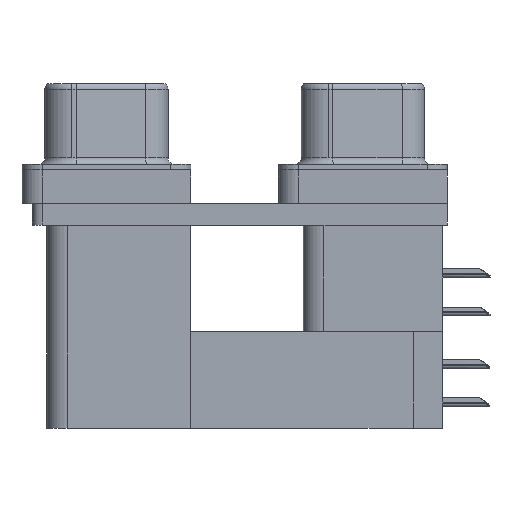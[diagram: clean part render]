
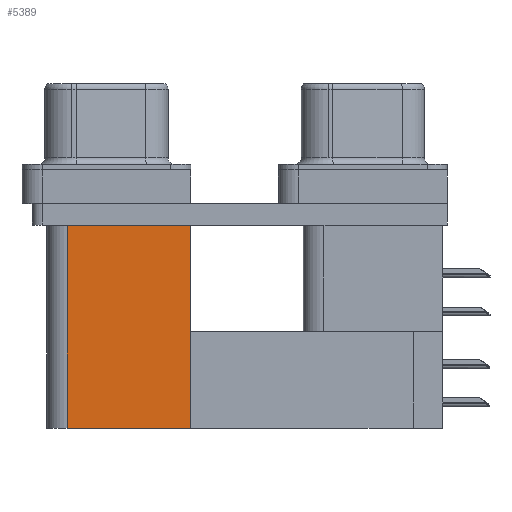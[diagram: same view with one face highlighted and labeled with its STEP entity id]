
A CAD part, left-side view. The second image highlights one B-rep face of the part: STEP entity #5389.
In plain terms, the highlighted planar face has unit normal (-1, 0, 0).
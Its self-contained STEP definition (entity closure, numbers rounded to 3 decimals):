
#396 = DIRECTION ( 'NONE',  ( 0., 1., 0. ) ) ;
#491 = PLANE ( 'NONE',  #10745 ) ;
#2394 = LINE ( 'NONE', #20965, #33138 ) ;
#3952 = ORIENTED_EDGE ( 'NONE', *, *, #31224, .F. ) ;
#5066 = FACE_OUTER_BOUND ( 'NONE', #18854, .T. ) ;
#5213 = VERTEX_POINT ( 'NONE', #20156 ) ;
#5389 = ADVANCED_FACE ( 'NONE', ( #5066 ), #491, .F. ) ;
#5781 = CARTESIAN_POINT ( 'NONE',  ( 3.7, 12.775, -19.2 ) ) ;
#6818 = ORIENTED_EDGE ( 'NONE', *, *, #19897, .T. ) ;
#6927 = CARTESIAN_POINT ( 'NONE',  ( 3.7, 21.975, -2.5 ) ) ;
#10745 = AXIS2_PLACEMENT_3D ( 'NONE', #29090, #12827, #19084 ) ;
#11218 = VECTOR ( 'NONE', #22201, 1000. ) ;
#12827 = DIRECTION ( 'NONE',  ( 1., 0., 0. ) ) ;
#14303 = DIRECTION ( 'NONE',  ( 0., 1., 0. ) ) ;
#15427 = CARTESIAN_POINT ( 'NONE',  ( 3.7, 21.975, -19.2 ) ) ;
#15797 = EDGE_CURVE ( 'NONE', #5213, #32626, #37083, .T. ) ;
#15876 = VECTOR ( 'NONE', #396, 1000. ) ;
#18787 = CARTESIAN_POINT ( 'NONE',  ( 3.7, 21.975, -19.2 ) ) ;
#18854 = EDGE_LOOP ( 'NONE', ( #6818, #21770, #3952, #30071 ) ) ;
#19084 = DIRECTION ( 'NONE',  ( 0., 1., 0. ) ) ;
#19897 = EDGE_CURVE ( 'NONE', #32626, #28933, #2394, .T. ) ;
#20156 = CARTESIAN_POINT ( 'NONE',  ( 3.7, 12.775, -19.2 ) ) ;
#20341 = EDGE_CURVE ( 'NONE', #39657, #28933, #33929, .T. ) ;
#20965 = CARTESIAN_POINT ( 'NONE',  ( 3.7, 12.775, -2.5 ) ) ;
#21770 = ORIENTED_EDGE ( 'NONE', *, *, #20341, .F. ) ;
#22201 = DIRECTION ( 'NONE',  ( 0., 0., 1. ) ) ;
#25040 = LINE ( 'NONE', #34527, #15876 ) ;
#25250 = CARTESIAN_POINT ( 'NONE',  ( 3.7, 12.775, -2.5 ) ) ;
#28933 = VERTEX_POINT ( 'NONE', #6927 ) ;
#29090 = CARTESIAN_POINT ( 'NONE',  ( 3.7, 12.775, -19.2 ) ) ;
#30071 = ORIENTED_EDGE ( 'NONE', *, *, #15797, .T. ) ;
#31224 = EDGE_CURVE ( 'NONE', #5213, #39657, #25040, .T. ) ;
#32626 = VERTEX_POINT ( 'NONE', #25250 ) ;
#33138 = VECTOR ( 'NONE', #14303, 1000. ) ;
#33458 = DIRECTION ( 'NONE',  ( 0., 0., 1. ) ) ;
#33929 = LINE ( 'NONE', #18787, #11218 ) ;
#34527 = CARTESIAN_POINT ( 'NONE',  ( 3.7, 12.775, -19.2 ) ) ;
#35464 = VECTOR ( 'NONE', #33458, 1000. ) ;
#37083 = LINE ( 'NONE', #5781, #35464 ) ;
#39657 = VERTEX_POINT ( 'NONE', #15427 ) ;
